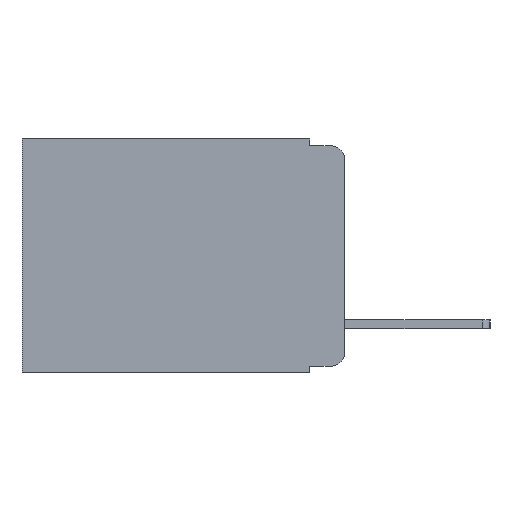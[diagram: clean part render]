
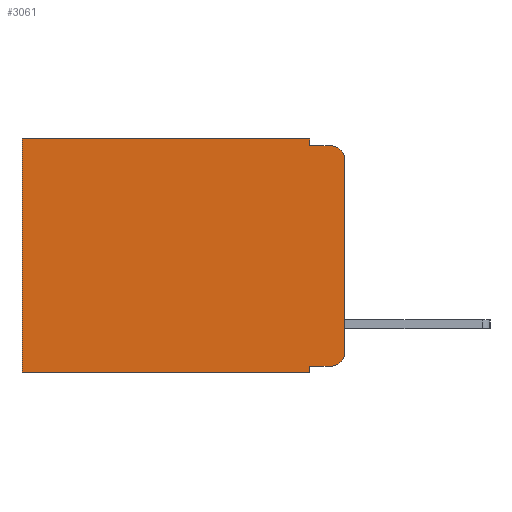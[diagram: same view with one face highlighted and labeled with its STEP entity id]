
A CAD part, left-side view. The second image highlights one B-rep face of the part: STEP entity #3061.
In plain terms, the highlighted planar face has unit normal (-1, 0, 0).
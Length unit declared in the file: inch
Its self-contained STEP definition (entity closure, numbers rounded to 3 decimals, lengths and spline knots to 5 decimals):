
#175 = VECTOR ( 'NONE', #10740, 39.37008 ) ;
#185 = DIRECTION ( 'NONE',  ( -1., 0., 0. ) ) ;
#530 = VECTOR ( 'NONE', #10216, 39.37008 ) ;
#723 = ORIENTED_EDGE ( 'NONE', *, *, #9497, .F. ) ;
#832 = VECTOR ( 'NONE', #12030, 39.37008 ) ;
#937 = ORIENTED_EDGE ( 'NONE', *, *, #13096, .T. ) ;
#1108 = EDGE_CURVE ( 'NONE', #2930, #6241, #11030, .T. ) ;
#1220 = ORIENTED_EDGE ( 'NONE', *, *, #7381, .F. ) ;
#1289 = EDGE_CURVE ( 'NONE', #12778, #2555, #8799, .T. ) ;
#1293 = CARTESIAN_POINT ( 'NONE',  ( 0.298, 0.473, 0. ) ) ;
#1821 = CIRCLE ( 'NONE', #2851, 0.02 ) ;
#1868 = EDGE_CURVE ( 'NONE', #2319, #3602, #13521, .T. ) ;
#2293 = ORIENTED_EDGE ( 'NONE', *, *, #1868, .F. ) ;
#2294 = ORIENTED_EDGE ( 'NONE', *, *, #8807, .T. ) ;
#2319 = VERTEX_POINT ( 'NONE', #3823 ) ;
#2422 = AXIS2_PLACEMENT_3D ( 'NONE', #9566, #3220, #10567 ) ;
#2555 = VERTEX_POINT ( 'NONE', #4303 ) ;
#2650 = VECTOR ( 'NONE', #7143, 39.37008 ) ;
#2796 = CARTESIAN_POINT ( 'NONE',  ( 0.298, 0., 0. ) ) ;
#2851 = AXIS2_PLACEMENT_3D ( 'NONE', #6653, #185, #7772 ) ;
#2930 = VERTEX_POINT ( 'NONE', #6834 ) ;
#2961 = CARTESIAN_POINT ( 'NONE',  ( 0.298, 0.051, -0.343 ) ) ;
#3061 = ADVANCED_FACE ( 'NONE', ( #9555 ), #7627, .F. ) ;
#3220 = DIRECTION ( 'NONE',  ( -1., 0., 0. ) ) ;
#3233 = VECTOR ( 'NONE', #5782, 39.37008 ) ;
#3419 = AXIS2_PLACEMENT_3D ( 'NONE', #7177, #8227, #4542 ) ;
#3602 = VERTEX_POINT ( 'NONE', #8599 ) ;
#3750 = VECTOR ( 'NONE', #4911, 39.37008 ) ;
#3823 = CARTESIAN_POINT ( 'NONE',  ( 0.298, 0.051, -0.01 ) ) ;
#4303 = CARTESIAN_POINT ( 'NONE',  ( 0.298, 0., -0.313 ) ) ;
#4406 = LINE ( 'NONE', #5814, #832 ) ;
#4542 = DIRECTION ( 'NONE',  ( 0., 0., -1. ) ) ;
#4705 = CARTESIAN_POINT ( 'NONE',  ( 0.298, 0.02, -0.333 ) ) ;
#4865 = CARTESIAN_POINT ( 'NONE',  ( 0.298, 0., -0.343 ) ) ;
#4911 = DIRECTION ( 'NONE',  ( 0., 1., 0. ) ) ;
#5782 = DIRECTION ( 'NONE',  ( 0., 1., 0. ) ) ;
#5814 = CARTESIAN_POINT ( 'NONE',  ( 0.298, 0.051, -0.333 ) ) ;
#5874 = DIRECTION ( 'NONE',  ( 0., 0., -1. ) ) ;
#6098 = EDGE_CURVE ( 'NONE', #10673, #2930, #8543, .T. ) ;
#6133 = ORIENTED_EDGE ( 'NONE', *, *, #6098, .T. ) ;
#6241 = VERTEX_POINT ( 'NONE', #11182 ) ;
#6441 = DIRECTION ( 'NONE',  ( 0., -1., 0. ) ) ;
#6595 = ORIENTED_EDGE ( 'NONE', *, *, #12555, .F. ) ;
#6653 = CARTESIAN_POINT ( 'NONE',  ( 0.298, 0.02, -0.313 ) ) ;
#6834 = CARTESIAN_POINT ( 'NONE',  ( 0.298, 0.473, 0. ) ) ;
#6864 = LINE ( 'NONE', #4865, #3750 ) ;
#7143 = DIRECTION ( 'NONE',  ( 0., 0., -1. ) ) ;
#7147 = ORIENTED_EDGE ( 'NONE', *, *, #1289, .F. ) ;
#7171 = VECTOR ( 'NONE', #5874, 39.37008 ) ;
#7177 = CARTESIAN_POINT ( 'NONE',  ( 0.298, 0., 0. ) ) ;
#7381 = EDGE_CURVE ( 'NONE', #10673, #2319, #12584, .T. ) ;
#7627 = PLANE ( 'NONE',  #3419 ) ;
#7772 = DIRECTION ( 'NONE',  ( 0., 0., -1. ) ) ;
#7787 = ORIENTED_EDGE ( 'NONE', *, *, #1108, .T. ) ;
#7899 = VERTEX_POINT ( 'NONE', #12845 ) ;
#8227 = DIRECTION ( 'NONE',  ( 1., 0., 0. ) ) ;
#8281 = VECTOR ( 'NONE', #6441, 39.37008 ) ;
#8543 = LINE ( 'NONE', #11991, #3233 ) ;
#8599 = CARTESIAN_POINT ( 'NONE',  ( 0.298, 0.02, -0.01 ) ) ;
#8645 = CARTESIAN_POINT ( 'NONE',  ( 0.298, 0.051, -0.01 ) ) ;
#8682 = ORIENTED_EDGE ( 'NONE', *, *, #8896, .T. ) ;
#8799 = LINE ( 'NONE', #2796, #175 ) ;
#8807 = EDGE_CURVE ( 'NONE', #12778, #3602, #9140, .T. ) ;
#8896 = EDGE_CURVE ( 'NONE', #10635, #2555, #1821, .T. ) ;
#9071 = CARTESIAN_POINT ( 'NONE',  ( 0.298, 0.051, 0. ) ) ;
#9117 = LINE ( 'NONE', #9200, #530 ) ;
#9140 = CIRCLE ( 'NONE', #2422, 0.02 ) ;
#9200 = CARTESIAN_POINT ( 'NONE',  ( 0.298, 0.051, 0. ) ) ;
#9352 = EDGE_LOOP ( 'NONE', ( #7147, #2294, #2293, #1220, #6133, #7787, #6595, #723, #937, #8682 ) ) ;
#9497 = EDGE_CURVE ( 'NONE', #7899, #9606, #9117, .T. ) ;
#9555 = FACE_OUTER_BOUND ( 'NONE', #9352, .T. ) ;
#9566 = CARTESIAN_POINT ( 'NONE',  ( 0.298, 0.02, -0.03 ) ) ;
#9606 = VERTEX_POINT ( 'NONE', #2961 ) ;
#10216 = DIRECTION ( 'NONE',  ( 0., 0., -1. ) ) ;
#10567 = DIRECTION ( 'NONE',  ( 0., 0., -1. ) ) ;
#10635 = VERTEX_POINT ( 'NONE', #4705 ) ;
#10673 = VERTEX_POINT ( 'NONE', #12955 ) ;
#10693 = CARTESIAN_POINT ( 'NONE',  ( 0.298, 0., -0.03 ) ) ;
#10740 = DIRECTION ( 'NONE',  ( 0., 0., -1. ) ) ;
#11030 = LINE ( 'NONE', #1293, #2650 ) ;
#11182 = CARTESIAN_POINT ( 'NONE',  ( 0.298, 0.473, -0.343 ) ) ;
#11991 = CARTESIAN_POINT ( 'NONE',  ( 0.298, 0., 0. ) ) ;
#12030 = DIRECTION ( 'NONE',  ( 0., -1., 0. ) ) ;
#12555 = EDGE_CURVE ( 'NONE', #9606, #6241, #6864, .T. ) ;
#12584 = LINE ( 'NONE', #9071, #7171 ) ;
#12778 = VERTEX_POINT ( 'NONE', #10693 ) ;
#12845 = CARTESIAN_POINT ( 'NONE',  ( 0.298, 0.051, -0.333 ) ) ;
#12955 = CARTESIAN_POINT ( 'NONE',  ( 0.298, 0.051, 0. ) ) ;
#13096 = EDGE_CURVE ( 'NONE', #7899, #10635, #4406, .T. ) ;
#13521 = LINE ( 'NONE', #8645, #8281 ) ;
